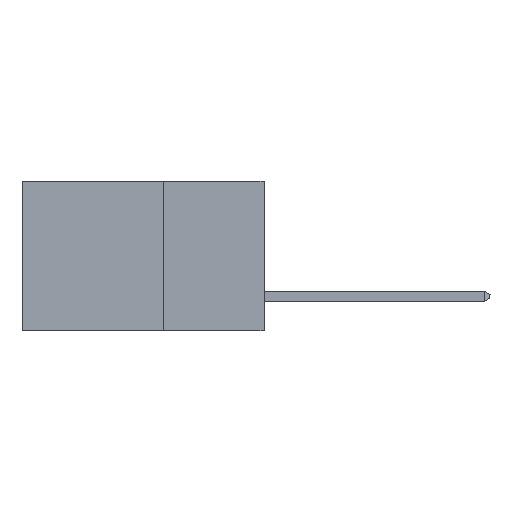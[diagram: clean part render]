
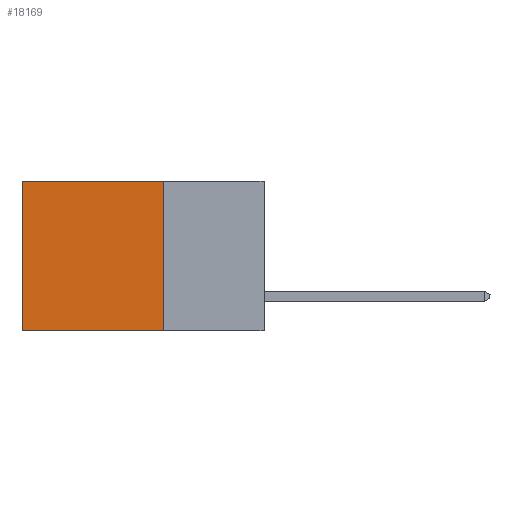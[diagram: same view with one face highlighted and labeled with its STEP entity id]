
A CAD part, left-side view. The second image highlights one B-rep face of the part: STEP entity #18169.
In plain terms, the highlighted planar face has unit normal (-1, 0, 0).
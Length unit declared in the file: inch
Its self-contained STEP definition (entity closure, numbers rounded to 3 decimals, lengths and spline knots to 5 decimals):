
#555 = LINE ( 'NONE', #4328, #4891 ) ;
#3242 = ORIENTED_EDGE ( 'NONE', *, *, #6473, .F. ) ;
#3263 = VECTOR ( 'NONE', #13694, 39.37008 ) ;
#3264 = VERTEX_POINT ( 'NONE', #10878 ) ;
#4328 = CARTESIAN_POINT ( 'NONE',  ( 0.2615, 0.25, -0.37 ) ) ;
#4378 = EDGE_LOOP ( 'NONE', ( #12487, #3242, #11095, #13221 ) ) ;
#4891 = VECTOR ( 'NONE', #9077, 39.37008 ) ;
#5135 = VECTOR ( 'NONE', #19988, 39.37008 ) ;
#5427 = DIRECTION ( 'NONE',  ( 0., 0., -1. ) ) ;
#5534 = FACE_OUTER_BOUND ( 'NONE', #4378, .T. ) ;
#6473 = EDGE_CURVE ( 'NONE', #20522, #3264, #555, .T. ) ;
#7836 = CARTESIAN_POINT ( 'NONE',  ( 0.2615, 0.25, -0.37 ) ) ;
#8056 = LINE ( 'NONE', #19646, #5135 ) ;
#8244 = VECTOR ( 'NONE', #12470, 39.37008 ) ;
#9077 = DIRECTION ( 'NONE',  ( 0., 1., 0. ) ) ;
#10452 = VERTEX_POINT ( 'NONE', #14563 ) ;
#10878 = CARTESIAN_POINT ( 'NONE',  ( 0.2615, 0.6, -0.37 ) ) ;
#11095 = ORIENTED_EDGE ( 'NONE', *, *, #17510, .F. ) ;
#11242 = EDGE_CURVE ( 'NONE', #12360, #10452, #13947, .T. ) ;
#11889 = CARTESIAN_POINT ( 'NONE',  ( 0.2615, 0.6, -0.37 ) ) ;
#12360 = VERTEX_POINT ( 'NONE', #13414 ) ;
#12470 = DIRECTION ( 'NONE',  ( 0., 1., 0. ) ) ;
#12487 = ORIENTED_EDGE ( 'NONE', *, *, #15550, .T. ) ;
#13221 = ORIENTED_EDGE ( 'NONE', *, *, #11242, .T. ) ;
#13414 = CARTESIAN_POINT ( 'NONE',  ( 0.2615, 0.25, 0. ) ) ;
#13471 = LINE ( 'NONE', #11889, #3263 ) ;
#13694 = DIRECTION ( 'NONE',  ( 0., 0., -1. ) ) ;
#13738 = CARTESIAN_POINT ( 'NONE',  ( 0.2615, 0.25, 0. ) ) ;
#13947 = LINE ( 'NONE', #13738, #8244 ) ;
#14137 = AXIS2_PLACEMENT_3D ( 'NONE', #17572, #19272, #5427 ) ;
#14563 = CARTESIAN_POINT ( 'NONE',  ( 0.2615, 0.6, 0. ) ) ;
#15550 = EDGE_CURVE ( 'NONE', #10452, #3264, #13471, .T. ) ;
#17510 = EDGE_CURVE ( 'NONE', #12360, #20522, #8056, .T. ) ;
#17572 = CARTESIAN_POINT ( 'NONE',  ( 0.2615, 0.25, -0.37 ) ) ;
#18169 = ADVANCED_FACE ( 'NONE', ( #5534 ), #20975, .F. ) ;
#19272 = DIRECTION ( 'NONE',  ( 1., 0., 0. ) ) ;
#19646 = CARTESIAN_POINT ( 'NONE',  ( 0.2615, 0.25, -0.37 ) ) ;
#19988 = DIRECTION ( 'NONE',  ( 0., 0., -1. ) ) ;
#20522 = VERTEX_POINT ( 'NONE', #7836 ) ;
#20975 = PLANE ( 'NONE',  #14137 ) ;
